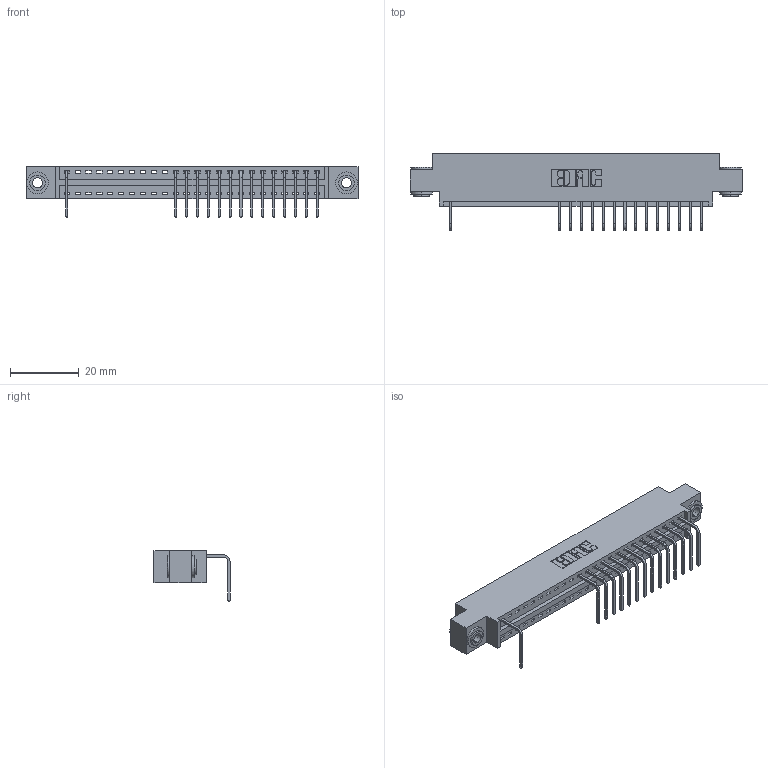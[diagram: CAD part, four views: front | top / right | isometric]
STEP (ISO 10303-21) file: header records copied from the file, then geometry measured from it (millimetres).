
FILE_DESCRIPTION (( 'STEP AP203' ), '1' );
FILE_NAME ('346-024-558-603.STEP', '2018-08-21T04:25:50', ( '' ), ( '' ), 'SwSTEP 2.0', 'SolidWorks 2016', '' );
FILE_SCHEMA (( 'CONFIG_CONTROL_DESIGN' ));
Length unit declared in the file: inch
Products named in the file (4): 345-250-002_345-250-002-102; 346-024-558-603; 346 Part_0.170 Offset - 0.156 Dia-TH; 345-292-001_558 Tail - 2
Assembly tree (18 placements, depth 2):
  346-024-558-603
    346 Part_0.170 Offset - 0.156 Dia-TH
    345-292-001_558 Tail - 2  x15
    345-250-002_345-250-002-102  x2
Bounding box: 96.77 x 22.16 x 14.73 mm (x, y, z)
Volume: 8951.2 mm3; surface area: 11117.5 mm2
Topology: 18 solids, 18 shells, 1172 faces, 3525 edges, 2326 vertices
Faces by surface type: plane 810, cylinder 354, cone 8
Entity records: 17896 total; most frequent: CARTESIAN_POINT 3094, ORIENTED_EDGE 3054, DIRECTION 2771, EDGE_CURVE 1527, LINE 1275, VECTOR 1275, VERTEX_POINT 1014, AXIS2_PLACEMENT_3D 748
